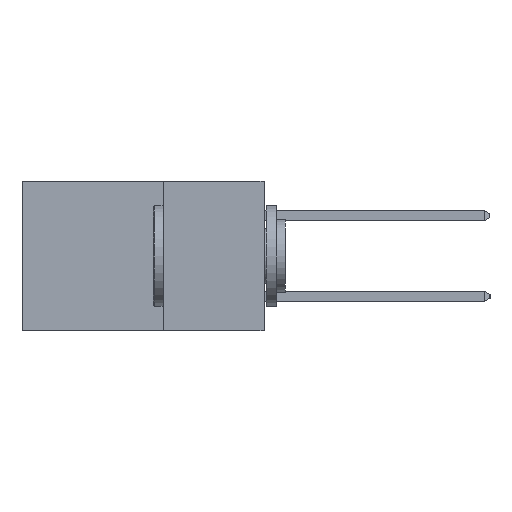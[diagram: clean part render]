
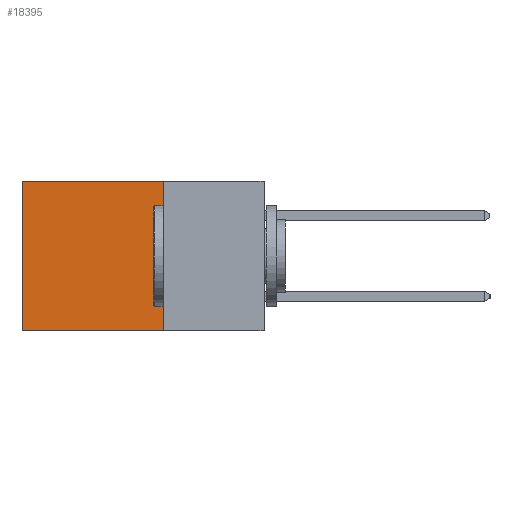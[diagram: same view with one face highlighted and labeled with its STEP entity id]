
A CAD part, left-side view. The second image highlights one B-rep face of the part: STEP entity #18395.
In plain terms, the highlighted planar face has unit normal (-1, 0, 0).
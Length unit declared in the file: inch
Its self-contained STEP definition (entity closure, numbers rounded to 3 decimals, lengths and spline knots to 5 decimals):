
#99 = CARTESIAN_POINT ( 'NONE',  ( 0.2615, 0.25, -0.37 ) ) ;
#360 = CARTESIAN_POINT ( 'NONE',  ( 0.2615, 0.25, 0. ) ) ;
#546 = EDGE_CURVE ( 'NONE', #14115, #15757, #21308, .T. ) ;
#2252 = DIRECTION ( 'NONE',  ( 0., 0., -1. ) ) ;
#2777 = ORIENTED_EDGE ( 'NONE', *, *, #2792, .T. ) ;
#2792 = EDGE_CURVE ( 'NONE', #15757, #6777, #20630, .T. ) ;
#2925 = AXIS2_PLACEMENT_3D ( 'NONE', #99, #14611, #2252 ) ;
#3978 = VERTEX_POINT ( 'NONE', #22251 ) ;
#5624 = DIRECTION ( 'NONE',  ( 0., 0., -1. ) ) ;
#6777 = VERTEX_POINT ( 'NONE', #15046 ) ;
#7319 = LINE ( 'NONE', #23609, #22648 ) ;
#7424 = EDGE_LOOP ( 'NONE', ( #2777, #23548, #19811, #22876 ) ) ;
#12575 = PLANE ( 'NONE',  #2925 ) ;
#12593 = VECTOR ( 'NONE', #14930, 39.37008 ) ;
#14115 = VERTEX_POINT ( 'NONE', #360 ) ;
#14611 = DIRECTION ( 'NONE',  ( 1., 0., 0. ) ) ;
#14930 = DIRECTION ( 'NONE',  ( 0., 1., 0. ) ) ;
#15046 = CARTESIAN_POINT ( 'NONE',  ( 0.2615, 0.6, -0.37 ) ) ;
#15757 = VERTEX_POINT ( 'NONE', #25902 ) ;
#15829 = DIRECTION ( 'NONE',  ( 0., 0., -1. ) ) ;
#16081 = VECTOR ( 'NONE', #20247, 39.37008 ) ;
#16276 = CARTESIAN_POINT ( 'NONE',  ( 0.2615, 0.6, -0.37 ) ) ;
#16608 = EDGE_CURVE ( 'NONE', #3978, #6777, #23089, .T. ) ;
#17444 = CARTESIAN_POINT ( 'NONE',  ( 0.2615, 0.25, 0. ) ) ;
#18395 = ADVANCED_FACE ( 'NONE', ( #22384 ), #12575, .F. ) ;
#19811 = ORIENTED_EDGE ( 'NONE', *, *, #23041, .F. ) ;
#20247 = DIRECTION ( 'NONE',  ( 0., 1., 0. ) ) ;
#20630 = LINE ( 'NONE', #16276, #21247 ) ;
#21247 = VECTOR ( 'NONE', #15829, 39.37008 ) ;
#21308 = LINE ( 'NONE', #17444, #16081 ) ;
#22251 = CARTESIAN_POINT ( 'NONE',  ( 0.2615, 0.25, -0.37 ) ) ;
#22384 = FACE_OUTER_BOUND ( 'NONE', #7424, .T. ) ;
#22648 = VECTOR ( 'NONE', #5624, 39.37008 ) ;
#22659 = CARTESIAN_POINT ( 'NONE',  ( 0.2615, 0.25, -0.37 ) ) ;
#22876 = ORIENTED_EDGE ( 'NONE', *, *, #546, .T. ) ;
#23041 = EDGE_CURVE ( 'NONE', #14115, #3978, #7319, .T. ) ;
#23089 = LINE ( 'NONE', #22659, #12593 ) ;
#23548 = ORIENTED_EDGE ( 'NONE', *, *, #16608, .F. ) ;
#23609 = CARTESIAN_POINT ( 'NONE',  ( 0.2615, 0.25, -0.37 ) ) ;
#25902 = CARTESIAN_POINT ( 'NONE',  ( 0.2615, 0.6, 0. ) ) ;
